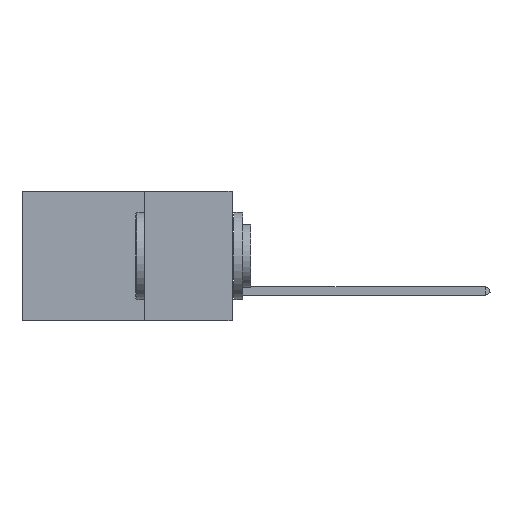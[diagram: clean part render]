
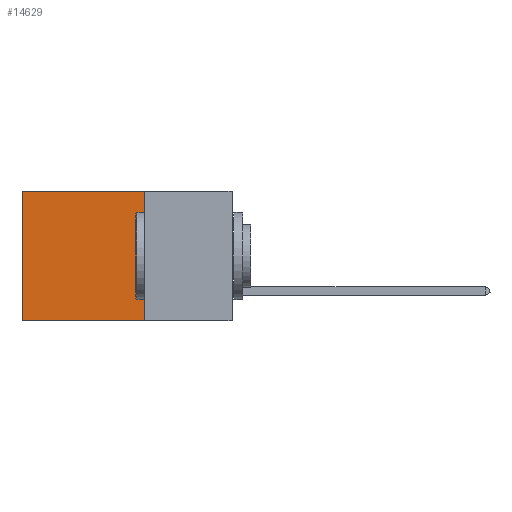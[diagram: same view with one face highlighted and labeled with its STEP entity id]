
A CAD part, left-side view. The second image highlights one B-rep face of the part: STEP entity #14629.
In plain terms, the highlighted planar face has unit normal (-1, 0, 0).
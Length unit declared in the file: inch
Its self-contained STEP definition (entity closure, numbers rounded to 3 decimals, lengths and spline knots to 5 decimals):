
#171 = LINE ( 'NONE', #4299, #21090 ) ;
#353 = VERTEX_POINT ( 'NONE', #22051 ) ;
#491 = DIRECTION ( 'NONE',  ( 0., 0., -1. ) ) ;
#545 = FACE_OUTER_BOUND ( 'NONE', #6303, .T. ) ;
#1142 = DIRECTION ( 'NONE',  ( 0., 0., -1. ) ) ;
#2389 = LINE ( 'NONE', #18644, #11339 ) ;
#3926 = DIRECTION ( 'NONE',  ( 0., 1., 0. ) ) ;
#4288 = AXIS2_PLACEMENT_3D ( 'NONE', #18032, #23382, #1142 ) ;
#4299 = CARTESIAN_POINT ( 'NONE',  ( 0.2875, 0.6, 0. ) ) ;
#4897 = CARTESIAN_POINT ( 'NONE',  ( 0.2875, 0.25, -0.37 ) ) ;
#5251 = VERTEX_POINT ( 'NONE', #4897 ) ;
#5371 = CARTESIAN_POINT ( 'NONE',  ( 0.2875, 0.25, 0. ) ) ;
#6117 = EDGE_CURVE ( 'NONE', #22786, #5251, #2389, .T. ) ;
#6303 = EDGE_LOOP ( 'NONE', ( #6561, #18514, #8185, #10312 ) ) ;
#6561 = ORIENTED_EDGE ( 'NONE', *, *, #10880, .T. ) ;
#6592 = DIRECTION ( 'NONE',  ( 0., 1., 0. ) ) ;
#6832 = PLANE ( 'NONE',  #4288 ) ;
#8185 = ORIENTED_EDGE ( 'NONE', *, *, #6117, .F. ) ;
#10312 = ORIENTED_EDGE ( 'NONE', *, *, #13672, .T. ) ;
#10880 = EDGE_CURVE ( 'NONE', #16201, #353, #171, .T. ) ;
#11339 = VECTOR ( 'NONE', #20208, 39.37008 ) ;
#13672 = EDGE_CURVE ( 'NONE', #22786, #16201, #22370, .T. ) ;
#14629 = ADVANCED_FACE ( 'NONE', ( #545 ), #6832, .F. ) ;
#14758 = EDGE_CURVE ( 'NONE', #5251, #353, #16494, .T. ) ;
#14881 = CARTESIAN_POINT ( 'NONE',  ( 0.2875, 0.25, 0. ) ) ;
#15895 = CARTESIAN_POINT ( 'NONE',  ( 0.2875, 0.25, -0.37 ) ) ;
#16201 = VERTEX_POINT ( 'NONE', #19251 ) ;
#16494 = LINE ( 'NONE', #15895, #22610 ) ;
#18032 = CARTESIAN_POINT ( 'NONE',  ( 0.2875, 0.25, 0. ) ) ;
#18514 = ORIENTED_EDGE ( 'NONE', *, *, #14758, .F. ) ;
#18644 = CARTESIAN_POINT ( 'NONE',  ( 0.2875, 0.25, 0. ) ) ;
#19251 = CARTESIAN_POINT ( 'NONE',  ( 0.2875, 0.6, 0. ) ) ;
#20208 = DIRECTION ( 'NONE',  ( 0., 0., -1. ) ) ;
#21090 = VECTOR ( 'NONE', #491, 39.37008 ) ;
#22051 = CARTESIAN_POINT ( 'NONE',  ( 0.2875, 0.6, -0.37 ) ) ;
#22370 = LINE ( 'NONE', #14881, #23227 ) ;
#22610 = VECTOR ( 'NONE', #6592, 39.37008 ) ;
#22786 = VERTEX_POINT ( 'NONE', #5371 ) ;
#23227 = VECTOR ( 'NONE', #3926, 39.37008 ) ;
#23382 = DIRECTION ( 'NONE',  ( 1., 0., 0. ) ) ;
